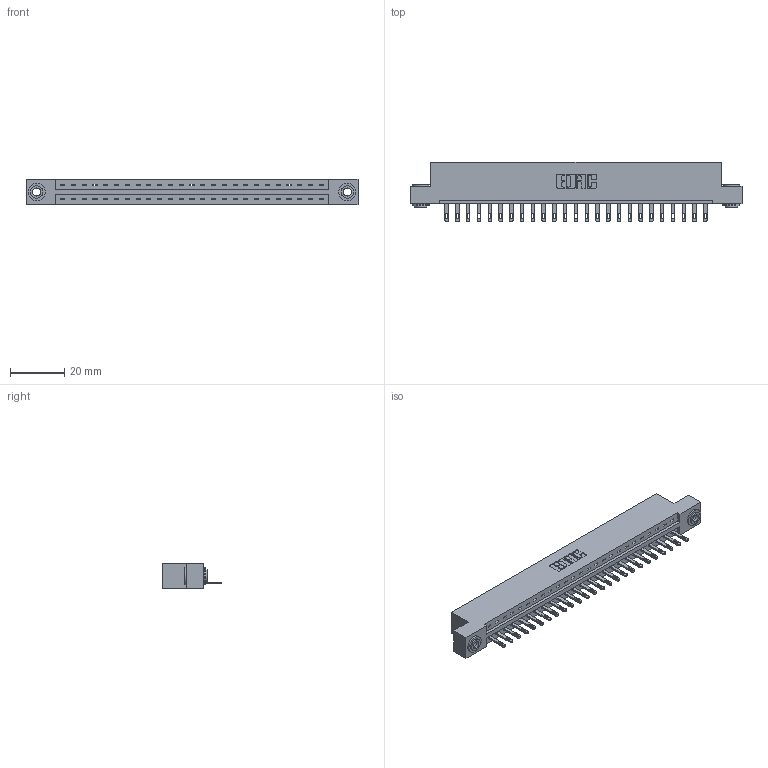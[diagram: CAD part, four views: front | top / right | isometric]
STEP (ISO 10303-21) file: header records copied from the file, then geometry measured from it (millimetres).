
FILE_DESCRIPTION (( 'STEP AP203' ), '1' );
FILE_NAME ('337-025-500-103.STEP', '2019-09-30T16:19:13', ( '' ), ( '' ), 'SwSTEP 2.0', 'SolidWorks 2016', '' );
FILE_SCHEMA (( 'CONFIG_CONTROL_DESIGN' ));
Length unit declared in the file: inch
Products named in the file (4): 337 Part_Flush Mounting Lugs - 0.156 Dia-TH; 337-025-500-103; 345-250-002_345-250-002-102; 345-292-001_345-293-100
Assembly tree (28 placements, depth 2):
  337-025-500-103
    337 Part_Flush Mounting Lugs - 0.156 Dia-TH
    345-292-001_345-293-100  x25
    345-250-002_345-250-002-102  x2
Bounding box: 122.07 x 21.85 x 9.4 mm (x, y, z)
Volume: 12509.5 mm3; surface area: 13123.5 mm2
Topology: 28 solids, 28 shells, 1602 faces, 4887 edges, 3254 vertices
Faces by surface type: plane 1080, cylinder 514, cone 8
Entity records: 21362 total; most frequent: CARTESIAN_POINT 3696, ORIENTED_EDGE 3650, DIRECTION 3181, EDGE_CURVE 1825, LINE 1669, VECTOR 1669, VERTEX_POINT 1214, AXIS2_PLACEMENT_3D 756
